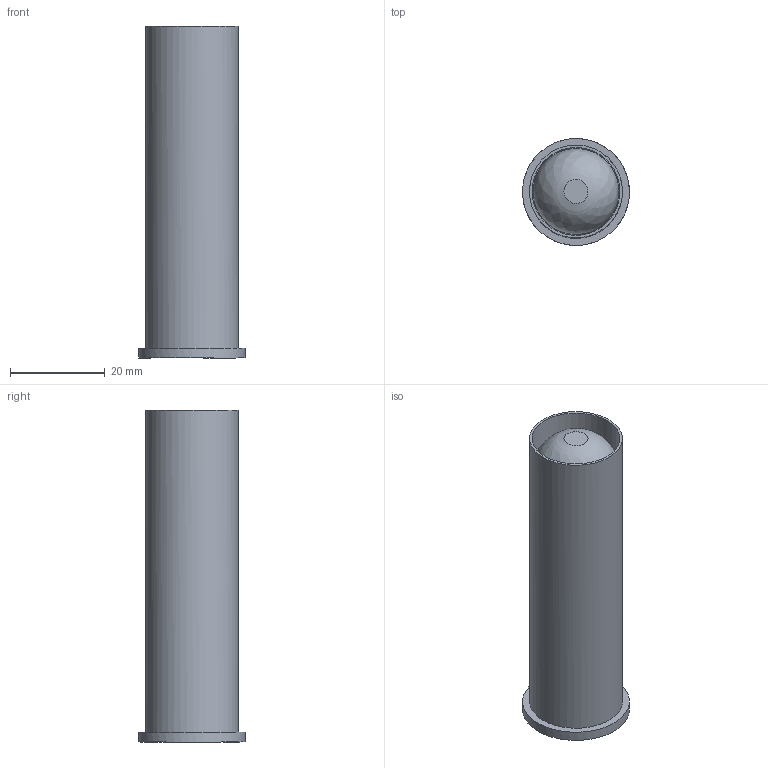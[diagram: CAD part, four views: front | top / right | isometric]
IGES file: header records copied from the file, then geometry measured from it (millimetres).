
Global section: file name: nessler air cartridge; native system: Autodesk Inventor 2017; preprocessor: unknown; author: user; date: 20201121.200057; units: millimetre
Bounding box: 22.5 x 22.5 x 69.9 mm (x, y, z)
Volume: 13948.9 mm3; surface area: 14931.5 mm2
Topology: 6 solids, 6 shells, 107 faces, 266 edges, 190 vertices
Faces by surface type: bspline 107
